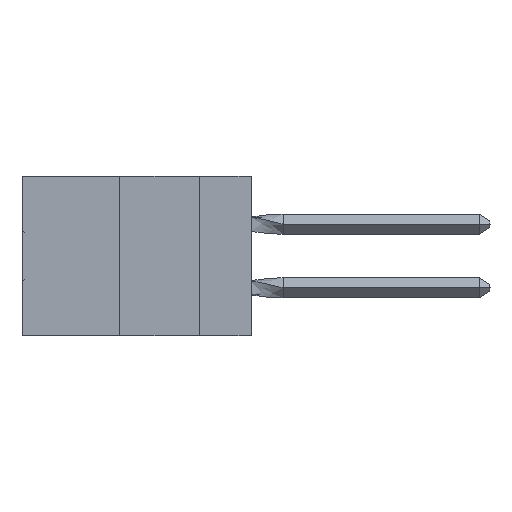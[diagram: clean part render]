
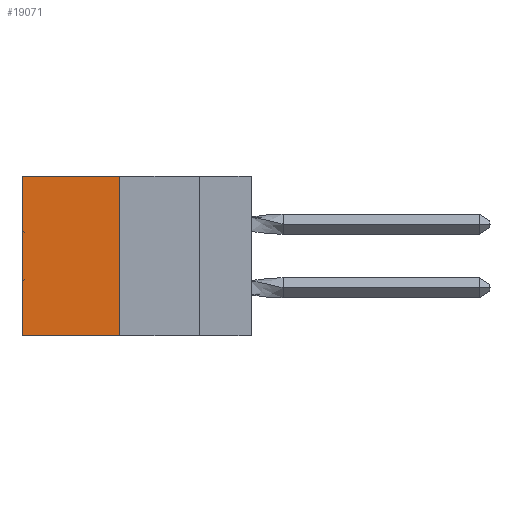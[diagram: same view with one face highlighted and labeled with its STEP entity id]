
A CAD part, left-side view. The second image highlights one B-rep face of the part: STEP entity #19071.
In plain terms, the highlighted planar face has unit normal (-1, 0, 0).
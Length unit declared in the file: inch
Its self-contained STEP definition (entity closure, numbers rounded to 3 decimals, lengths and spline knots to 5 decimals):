
#1197 = EDGE_CURVE ( 'NONE', #36745, #14727, #2243, .T. ) ;
#1519 = ORIENTED_EDGE ( 'NONE', *, *, #30622, .T. ) ;
#1662 = LINE ( 'NONE', #2156, #32966 ) ;
#2156 = CARTESIAN_POINT ( 'NONE',  ( 0.305, 0.413, -0.5 ) ) ;
#2243 = LINE ( 'NONE', #6648, #41963 ) ;
#3119 = VECTOR ( 'NONE', #18877, 39.37008 ) ;
#3730 = CARTESIAN_POINT ( 'NONE',  ( 0.305, 0.72, -0.5 ) ) ;
#5841 = CARTESIAN_POINT ( 'NONE',  ( 0.305, 0.413, 0. ) ) ;
#6222 = CARTESIAN_POINT ( 'NONE',  ( 0.305, 0.72, -0.5 ) ) ;
#6648 = CARTESIAN_POINT ( 'NONE',  ( 0.305, 0.413, -0.5 ) ) ;
#6706 = VERTEX_POINT ( 'NONE', #6222 ) ;
#10117 = DIRECTION ( 'NONE',  ( 0., 1., 0. ) ) ;
#10496 = CARTESIAN_POINT ( 'NONE',  ( 0.305, 0.413, 0. ) ) ;
#10928 = DIRECTION ( 'NONE',  ( 1., 0., 0. ) ) ;
#12916 = ORIENTED_EDGE ( 'NONE', *, *, #1197, .F. ) ;
#14568 = AXIS2_PLACEMENT_3D ( 'NONE', #43333, #10928, #40472 ) ;
#14727 = VERTEX_POINT ( 'NONE', #23458 ) ;
#16213 = CARTESIAN_POINT ( 'NONE',  ( 0.305, 0.72, 0. ) ) ;
#16306 = ORIENTED_EDGE ( 'NONE', *, *, #19255, .T. ) ;
#18877 = DIRECTION ( 'NONE',  ( 0., 0., -1. ) ) ;
#19071 = ADVANCED_FACE ( 'NONE', ( #44097 ), #35212, .F. ) ;
#19255 = EDGE_CURVE ( 'NONE', #19321, #6706, #24815, .T. ) ;
#19321 = VERTEX_POINT ( 'NONE', #16213 ) ;
#23458 = CARTESIAN_POINT ( 'NONE',  ( 0.305, 0.413, -0.5 ) ) ;
#24815 = LINE ( 'NONE', #3730, #3119 ) ;
#26652 = DIRECTION ( 'NONE',  ( 0., 0., -1. ) ) ;
#30622 = EDGE_CURVE ( 'NONE', #36745, #19321, #47291, .T. ) ;
#31794 = DIRECTION ( 'NONE',  ( 0., 1., 0. ) ) ;
#31854 = EDGE_CURVE ( 'NONE', #14727, #6706, #1662, .T. ) ;
#32966 = VECTOR ( 'NONE', #31794, 39.37008 ) ;
#35212 = PLANE ( 'NONE',  #14568 ) ;
#36745 = VERTEX_POINT ( 'NONE', #10496 ) ;
#40466 = ORIENTED_EDGE ( 'NONE', *, *, #31854, .F. ) ;
#40472 = DIRECTION ( 'NONE',  ( 0., 0., -1. ) ) ;
#40844 = EDGE_LOOP ( 'NONE', ( #16306, #40466, #12916, #1519 ) ) ;
#41963 = VECTOR ( 'NONE', #26652, 39.37008 ) ;
#43333 = CARTESIAN_POINT ( 'NONE',  ( 0.305, 0.413, -0.5 ) ) ;
#44097 = FACE_OUTER_BOUND ( 'NONE', #40844, .T. ) ;
#45987 = VECTOR ( 'NONE', #10117, 39.37008 ) ;
#47291 = LINE ( 'NONE', #5841, #45987 ) ;
